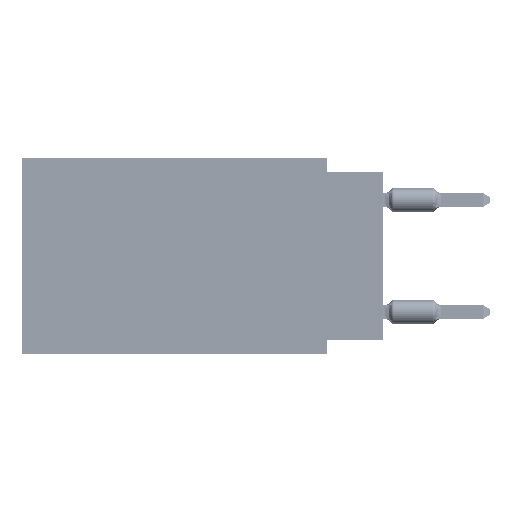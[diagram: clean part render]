
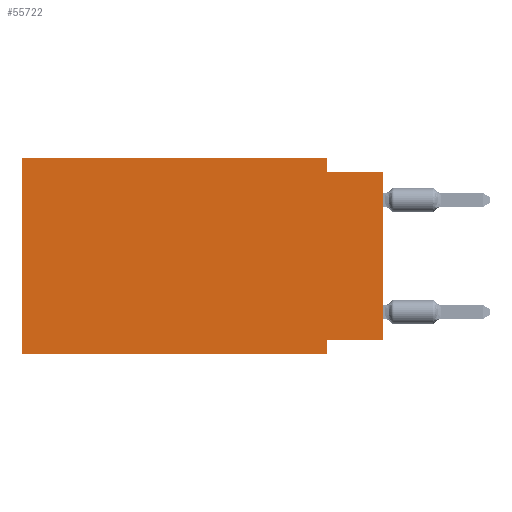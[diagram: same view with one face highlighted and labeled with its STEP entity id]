
A CAD part, left-side view. The second image highlights one B-rep face of the part: STEP entity #55722.
In plain terms, the highlighted planar face has unit normal (-1, 0, 0).
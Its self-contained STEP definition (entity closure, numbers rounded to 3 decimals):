
#299 = CARTESIAN_POINT ( 'NONE',  ( 0., 2.54, 0. ) ) ;
#754 = ORIENTED_EDGE ( 'NONE', *, *, #54105, .T. ) ;
#1559 = VERTEX_POINT ( 'NONE', #4141 ) ;
#3001 = DIRECTION ( 'NONE',  ( 0., 0., 1. ) ) ;
#3172 = VERTEX_POINT ( 'NONE', #299 ) ;
#4141 = CARTESIAN_POINT ( 'NONE',  ( 0., 16.383, 0. ) ) ;
#4813 = CARTESIAN_POINT ( 'NONE',  ( 0., 2.54, 0. ) ) ;
#4842 = DIRECTION ( 'NONE',  ( 0., -1., 0. ) ) ;
#5177 = CARTESIAN_POINT ( 'NONE',  ( 0., 0., -8.255 ) ) ;
#5397 = VECTOR ( 'NONE', #41443, 1000. ) ;
#7648 = CARTESIAN_POINT ( 'NONE',  ( 0., 16.383, 0. ) ) ;
#10898 = CARTESIAN_POINT ( 'NONE',  ( 0., 0., -8.255 ) ) ;
#10944 = CARTESIAN_POINT ( 'NONE',  ( 0., 2.54, -8.89 ) ) ;
#11375 = CARTESIAN_POINT ( 'NONE',  ( 0., 16.383, -8.89 ) ) ;
#14231 = VECTOR ( 'NONE', #54899, 1000. ) ;
#18598 = FACE_OUTER_BOUND ( 'NONE', #37951, .T. ) ;
#18629 = CARTESIAN_POINT ( 'NONE',  ( 0., 2.54, -8.89 ) ) ;
#19297 = VERTEX_POINT ( 'NONE', #5177 ) ;
#19347 = LINE ( 'NONE', #35417, #30708 ) ;
#20068 = CARTESIAN_POINT ( 'NONE',  ( 0., 16.383, 0. ) ) ;
#20257 = CARTESIAN_POINT ( 'NONE',  ( 0., 0., -0.635 ) ) ;
#20507 = CARTESIAN_POINT ( 'NONE',  ( 0., 0., -0.635 ) ) ;
#20757 = ORIENTED_EDGE ( 'NONE', *, *, #66746, .F. ) ;
#21140 = ORIENTED_EDGE ( 'NONE', *, *, #52076, .F. ) ;
#22450 = ORIENTED_EDGE ( 'NONE', *, *, #38130, .F. ) ;
#24069 = DIRECTION ( 'NONE',  ( 1., 0., 0. ) ) ;
#25219 = VERTEX_POINT ( 'NONE', #10944 ) ;
#25544 = DIRECTION ( 'NONE',  ( 0., -1., 0. ) ) ;
#28350 = CARTESIAN_POINT ( 'NONE',  ( 0., 16.383, -8.89 ) ) ;
#29201 = EDGE_CURVE ( 'NONE', #46866, #25219, #42864, .T. ) ;
#30368 = LINE ( 'NONE', #20068, #41684 ) ;
#30706 = VECTOR ( 'NONE', #3001, 1000. ) ;
#30708 = VECTOR ( 'NONE', #34414, 1000. ) ;
#31452 = DIRECTION ( 'NONE',  ( 0., 1., 0. ) ) ;
#34011 = PLANE ( 'NONE',  #36176 ) ;
#34414 = DIRECTION ( 'NONE',  ( 0., 0., 1. ) ) ;
#35417 = CARTESIAN_POINT ( 'NONE',  ( 0., 16.383, 0. ) ) ;
#35648 = LINE ( 'NONE', #4813, #5397 ) ;
#36176 = AXIS2_PLACEMENT_3D ( 'NONE', #7648, #24069, #39808 ) ;
#37258 = LINE ( 'NONE', #10898, #55762 ) ;
#37622 = VECTOR ( 'NONE', #47654, 1000. ) ;
#37951 = EDGE_LOOP ( 'NONE', ( #754, #54274, #21140, #57320, #22450, #62493, #20757, #43531 ) ) ;
#38130 = EDGE_CURVE ( 'NONE', #46866, #1559, #19347, .T. ) ;
#39808 = DIRECTION ( 'NONE',  ( 0., 0., -1. ) ) ;
#41443 = DIRECTION ( 'NONE',  ( 0., 0., -1. ) ) ;
#41684 = VECTOR ( 'NONE', #25544, 1000. ) ;
#42864 = LINE ( 'NONE', #11375, #37622 ) ;
#43531 = ORIENTED_EDGE ( 'NONE', *, *, #52637, .F. ) ;
#46257 = LINE ( 'NONE', #20257, #49728 ) ;
#46351 = EDGE_CURVE ( 'NONE', #65920, #61436, #46257, .T. ) ;
#46866 = VERTEX_POINT ( 'NONE', #28350 ) ;
#47654 = DIRECTION ( 'NONE',  ( 0., -1., 0. ) ) ;
#48676 = CARTESIAN_POINT ( 'NONE',  ( 0., 2.54, -8.255 ) ) ;
#49728 = VECTOR ( 'NONE', #4842, 1000. ) ;
#50513 = CARTESIAN_POINT ( 'NONE',  ( 0., 2.54, -0.635 ) ) ;
#52076 = EDGE_CURVE ( 'NONE', #3172, #65920, #35648, .T. ) ;
#52637 = EDGE_CURVE ( 'NONE', #19297, #67014, #37258, .T. ) ;
#54105 = EDGE_CURVE ( 'NONE', #19297, #61436, #58820, .T. ) ;
#54242 = EDGE_CURVE ( 'NONE', #1559, #3172, #30368, .T. ) ;
#54274 = ORIENTED_EDGE ( 'NONE', *, *, #46351, .F. ) ;
#54899 = DIRECTION ( 'NONE',  ( 0., 0., -1. ) ) ;
#55583 = LINE ( 'NONE', #18629, #14231 ) ;
#55722 = ADVANCED_FACE ( 'NONE', ( #18598 ), #34011, .F. ) ;
#55762 = VECTOR ( 'NONE', #31452, 1000. ) ;
#57320 = ORIENTED_EDGE ( 'NONE', *, *, #54242, .F. ) ;
#58820 = LINE ( 'NONE', #59471, #30706 ) ;
#59471 = CARTESIAN_POINT ( 'NONE',  ( 0., 0., 0. ) ) ;
#61436 = VERTEX_POINT ( 'NONE', #20507 ) ;
#62493 = ORIENTED_EDGE ( 'NONE', *, *, #29201, .T. ) ;
#65920 = VERTEX_POINT ( 'NONE', #50513 ) ;
#66746 = EDGE_CURVE ( 'NONE', #67014, #25219, #55583, .T. ) ;
#67014 = VERTEX_POINT ( 'NONE', #48676 ) ;
